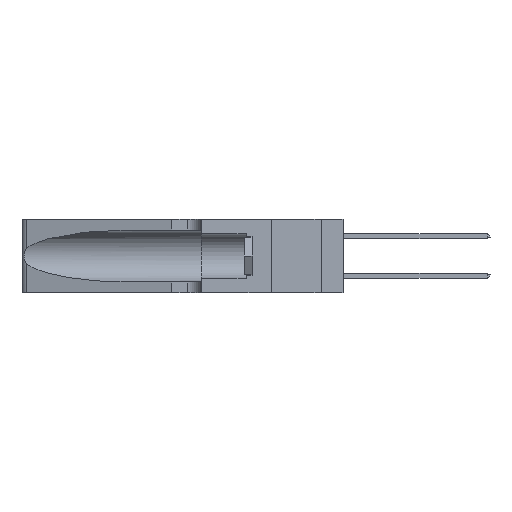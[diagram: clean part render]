
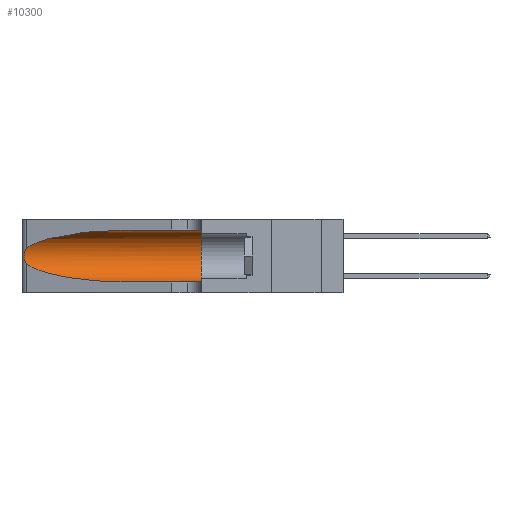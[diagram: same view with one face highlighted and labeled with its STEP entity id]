
A CAD part, left-side view. The second image highlights one B-rep face of the part: STEP entity #10300.
In plain terms, the highlighted cylindrical face has radius 3.308 mm (diameter 6.617 mm), a partial arc.
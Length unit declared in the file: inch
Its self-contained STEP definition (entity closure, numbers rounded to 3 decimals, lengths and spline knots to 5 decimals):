
#664 = CARTESIAN_POINT ( 'NONE',  ( 0.1305, 0.35, 0.05475 ) ) ;
#1780 = CARTESIAN_POINT ( 'NONE',  ( 0.25487, 1.22718, 0.22369 ) ) ;
#1839 = CARTESIAN_POINT ( 'NONE',  ( 0.25487, 1.22718, 0.22369 ) ) ;
#1945 = CARTESIAN_POINT ( 'NONE',  ( 0.26075, 1.23896, 0.178 ) ) ;
#1999 = LINE ( 'NONE', #14735, #18983 ) ;
#2492 = CARTESIAN_POINT ( 'NONE',  ( 0.18966, 0.96281, 0.05475 ) ) ;
#2602 = DIRECTION ( 'NONE',  ( 0., -1., 0. ) ) ;
#3340 = ORIENTED_EDGE ( 'NONE', *, *, #28440, .F. ) ;
#3780 = B_SPLINE_CURVE_WITH_KNOTS ( 'NONE', 3,
 ( #1839, #23346, #11683, #27983, #14112, #30276, #16508, #1945, #18838, #4440, #21160, #6885, #23449, #9335 ),
 .UNSPECIFIED., .F., .F.,
 ( 4, 2, 2, 2, 2, 2, 4 ),
 ( 0., 0.00027, 0.00053, 0.00107, 0.0016, 0.00187, 0.00214 ),
 .UNSPECIFIED. ) ;
#4114 = LINE ( 'NONE', #19398, #9825 ) ;
#4440 = CARTESIAN_POINT ( 'NONE',  ( 0.25856, 1.23593, 0.16098 ) ) ;
#4648 = ORIENTED_EDGE ( 'NONE', *, *, #11397, .T. ) ;
#4828 =( BOUNDED_CURVE ( )  B_SPLINE_CURVE ( 3, ( #23851, #14628, #2492, #19348 ),
 .UNSPECIFIED., .F., .T. ) 
 B_SPLINE_CURVE_WITH_KNOTS ( ( 4, 4 ),
 ( 3.44316, 4.71239 ),
 .UNSPECIFIED. ) 
 CURVE ( )  GEOMETRIC_REPRESENTATION_ITEM ( )  RATIONAL_B_SPLINE_CURVE ( ( 1., 0.87, 0.87, 1. ) ) 
 REPRESENTATION_ITEM ( '' )  );
#5599 = CARTESIAN_POINT ( 'NONE',  ( 0.1305, 1.61858, 0.185 ) ) ;
#5706 = DIRECTION ( 'NONE',  ( 0., -1., 0. ) ) ;
#6885 = CARTESIAN_POINT ( 'NONE',  ( 0.25639, 1.23186, 0.15144 ) ) ;
#6946 = CARTESIAN_POINT ( 'NONE',  ( 0.1305, 0.72297, 0.05475 ) ) ;
#7155 =( BOUNDED_CURVE ( )  B_SPLINE_CURVE ( 3, ( #9589, #23693, #12028, #28324 ),
 .UNSPECIFIED., .F., .F. ) 
 B_SPLINE_CURVE_WITH_KNOTS ( ( 4, 4 ),
 ( 1.5708, 2.84003 ),
 .UNSPECIFIED. ) 
 CURVE ( )  GEOMETRIC_REPRESENTATION_ITEM ( )  RATIONAL_B_SPLINE_CURVE ( ( 1., 0.87, 0.87, 1. ) ) 
 REPRESENTATION_ITEM ( '' )  );
#7695 = ORIENTED_EDGE ( 'NONE', *, *, #22667, .T. ) ;
#8532 = EDGE_CURVE ( 'NONE', #22291, #14432, #11499, .T. ) ;
#8997 = CARTESIAN_POINT ( 'NONE',  ( 0.1305, 0.35, 0.185 ) ) ;
#9335 = CARTESIAN_POINT ( 'NONE',  ( 0.25487, 1.22718, 0.14631 ) ) ;
#9416 = VERTEX_POINT ( 'NONE', #30589 ) ;
#9589 = CARTESIAN_POINT ( 'NONE',  ( 0.1305, 0.72297, 0.31525 ) ) ;
#9825 = VECTOR ( 'NONE', #28533, 39.37008 ) ;
#10300 = ADVANCED_FACE ( 'NONE', ( #24436 ), #17613, .F. ) ;
#10510 = ORIENTED_EDGE ( 'NONE', *, *, #11626, .T. ) ;
#11397 = EDGE_CURVE ( 'NONE', #9416, #24443, #7155, .T. ) ;
#11457 = DIRECTION ( 'NONE',  ( 0., 0., 1. ) ) ;
#11499 = CIRCLE ( 'NONE', #23777, 0.13025 ) ;
#11626 = EDGE_CURVE ( 'NONE', #26330, #14432, #1999, .T. ) ;
#11683 = CARTESIAN_POINT ( 'NONE',  ( 0.25639, 1.23184, 0.21858 ) ) ;
#11736 = ORIENTED_EDGE ( 'NONE', *, *, #25619, .T. ) ;
#12028 = CARTESIAN_POINT ( 'NONE',  ( 0.2373, 1.15595, 0.28018 ) ) ;
#14112 = CARTESIAN_POINT ( 'NONE',  ( 0.25854, 1.2359, 0.20912 ) ) ;
#14432 = VERTEX_POINT ( 'NONE', #664 ) ;
#14628 = CARTESIAN_POINT ( 'NONE',  ( 0.2373, 1.15595, 0.08982 ) ) ;
#14735 = CARTESIAN_POINT ( 'NONE',  ( 0.1305, 1.61858, 0.05475 ) ) ;
#16508 = CARTESIAN_POINT ( 'NONE',  ( 0.26075, 1.23896, 0.19203 ) ) ;
#17613 = CYLINDRICAL_SURFACE ( 'NONE', #17847, 0.13025 ) ;
#17847 = AXIS2_PLACEMENT_3D ( 'NONE', #5599, #5706, #20060 ) ;
#18838 = CARTESIAN_POINT ( 'NONE',  ( 0.26017, 1.23833, 0.17102 ) ) ;
#18983 = VECTOR ( 'NONE', #2602, 39.37008 ) ;
#19348 = CARTESIAN_POINT ( 'NONE',  ( 0.1305, 0.72297, 0.05475 ) ) ;
#19398 = CARTESIAN_POINT ( 'NONE',  ( 0.1305, 1.61858, 0.31525 ) ) ;
#20060 = DIRECTION ( 'NONE',  ( 0., 0., -1. ) ) ;
#20377 = CARTESIAN_POINT ( 'NONE',  ( 0.1305, 0.35, 0.31525 ) ) ;
#20594 = VERTEX_POINT ( 'NONE', #30181 ) ;
#21160 = CARTESIAN_POINT ( 'NONE',  ( 0.25789, 1.23486, 0.15765 ) ) ;
#22291 = VERTEX_POINT ( 'NONE', #20377 ) ;
#22667 = EDGE_CURVE ( 'NONE', #20594, #26330, #4828, .T. ) ;
#23346 = CARTESIAN_POINT ( 'NONE',  ( 0.25555, 1.22994, 0.2215 ) ) ;
#23449 = CARTESIAN_POINT ( 'NONE',  ( 0.25555, 1.22993, 0.14849 ) ) ;
#23693 = CARTESIAN_POINT ( 'NONE',  ( 0.18966, 0.96281, 0.31525 ) ) ;
#23777 = AXIS2_PLACEMENT_3D ( 'NONE', #8997, #25464, #11457 ) ;
#23851 = CARTESIAN_POINT ( 'NONE',  ( 0.25487, 1.22718, 0.14631 ) ) ;
#24436 = FACE_OUTER_BOUND ( 'NONE', #26771, .T. ) ;
#24443 = VERTEX_POINT ( 'NONE', #1780 ) ;
#25464 = DIRECTION ( 'NONE',  ( 0., 1., 0. ) ) ;
#25619 = EDGE_CURVE ( 'NONE', #24443, #20594, #3780, .T. ) ;
#26330 = VERTEX_POINT ( 'NONE', #6946 ) ;
#26771 = EDGE_LOOP ( 'NONE', ( #4648, #11736, #7695, #10510, #28348, #3340 ) ) ;
#27983 = CARTESIAN_POINT ( 'NONE',  ( 0.25787, 1.23484, 0.2124 ) ) ;
#28324 = CARTESIAN_POINT ( 'NONE',  ( 0.25487, 1.22718, 0.22369 ) ) ;
#28348 = ORIENTED_EDGE ( 'NONE', *, *, #8532, .F. ) ;
#28440 = EDGE_CURVE ( 'NONE', #9416, #22291, #4114, .T. ) ;
#28533 = DIRECTION ( 'NONE',  ( 0., -1., 0. ) ) ;
#30181 = CARTESIAN_POINT ( 'NONE',  ( 0.25487, 1.22718, 0.14631 ) ) ;
#30276 = CARTESIAN_POINT ( 'NONE',  ( 0.26018, 1.23835, 0.19895 ) ) ;
#30589 = CARTESIAN_POINT ( 'NONE',  ( 0.1305, 0.72297, 0.31525 ) ) ;
